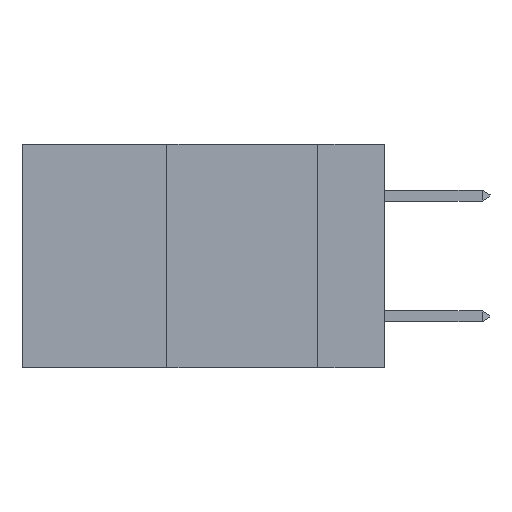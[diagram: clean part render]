
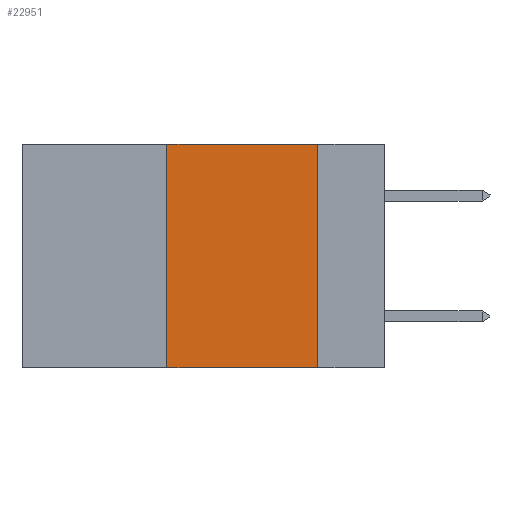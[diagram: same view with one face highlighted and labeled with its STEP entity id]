
A CAD part, left-side view. The second image highlights one B-rep face of the part: STEP entity #22951.
In plain terms, the highlighted planar face has unit normal (-1, 0, 0).
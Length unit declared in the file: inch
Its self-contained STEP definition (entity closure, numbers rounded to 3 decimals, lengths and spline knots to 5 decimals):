
#776 = DIRECTION ( 'NONE',  ( 1., 0., 0. ) ) ;
#3693 = CARTESIAN_POINT ( 'NONE',  ( 0., 0.11, -0.37 ) ) ;
#3780 = EDGE_CURVE ( 'NONE', #7527, #15951, #7805, .T. ) ;
#4807 = LINE ( 'NONE', #9633, #33023 ) ;
#4959 = CARTESIAN_POINT ( 'NONE',  ( 0., 0.6, -0.37 ) ) ;
#5846 = VERTEX_POINT ( 'NONE', #14678 ) ;
#6354 = VECTOR ( 'NONE', #13246, 39.37008 ) ;
#7527 = VERTEX_POINT ( 'NONE', #26987 ) ;
#7805 = LINE ( 'NONE', #25422, #17077 ) ;
#8479 = DIRECTION ( 'NONE',  ( 0., 0., -1. ) ) ;
#8968 = VERTEX_POINT ( 'NONE', #24429 ) ;
#9152 = PLANE ( 'NONE',  #14253 ) ;
#9633 = CARTESIAN_POINT ( 'NONE',  ( 0., 0.6, 0. ) ) ;
#12015 = ORIENTED_EDGE ( 'NONE', *, *, #26069, .F. ) ;
#12041 = FACE_OUTER_BOUND ( 'NONE', #22315, .T. ) ;
#13246 = DIRECTION ( 'NONE',  ( 0., 0., 1. ) ) ;
#13424 = DIRECTION ( 'NONE',  ( 0., -1., 0. ) ) ;
#14253 = AXIS2_PLACEMENT_3D ( 'NONE', #26094, #776, #20531 ) ;
#14678 = CARTESIAN_POINT ( 'NONE',  ( 0., 0.36, 0. ) ) ;
#15951 = VERTEX_POINT ( 'NONE', #3693 ) ;
#17077 = VECTOR ( 'NONE', #8479, 39.37008 ) ;
#17792 = ORIENTED_EDGE ( 'NONE', *, *, #3780, .F. ) ;
#19619 = VECTOR ( 'NONE', #13424, 39.37008 ) ;
#20531 = DIRECTION ( 'NONE',  ( 0., 0., -1. ) ) ;
#21322 = ORIENTED_EDGE ( 'NONE', *, *, #36068, .T. ) ;
#22315 = EDGE_LOOP ( 'NONE', ( #17792, #12015, #34532, #21322 ) ) ;
#22951 = ADVANCED_FACE ( 'NONE', ( #12041 ), #9152, .F. ) ;
#24429 = CARTESIAN_POINT ( 'NONE',  ( 0., 0.36, -0.37 ) ) ;
#25422 = CARTESIAN_POINT ( 'NONE',  ( 0., 0.11, 0. ) ) ;
#26069 = EDGE_CURVE ( 'NONE', #5846, #7527, #4807, .T. ) ;
#26094 = CARTESIAN_POINT ( 'NONE',  ( 0., 0.6, 0. ) ) ;
#26987 = CARTESIAN_POINT ( 'NONE',  ( 0., 0.11, 0. ) ) ;
#27126 = LINE ( 'NONE', #4959, #19619 ) ;
#28852 = LINE ( 'NONE', #30153, #6354 ) ;
#29034 = EDGE_CURVE ( 'NONE', #8968, #5846, #28852, .T. ) ;
#29375 = DIRECTION ( 'NONE',  ( 0., -1., 0. ) ) ;
#30153 = CARTESIAN_POINT ( 'NONE',  ( 0., 0.36, 0. ) ) ;
#33023 = VECTOR ( 'NONE', #29375, 39.37008 ) ;
#34532 = ORIENTED_EDGE ( 'NONE', *, *, #29034, .F. ) ;
#36068 = EDGE_CURVE ( 'NONE', #8968, #15951, #27126, .T. ) ;
